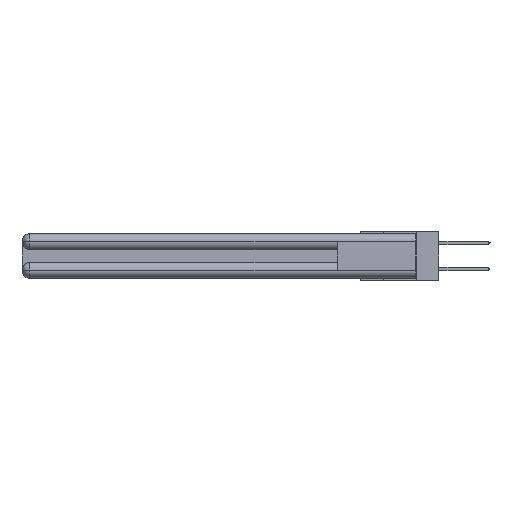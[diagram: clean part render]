
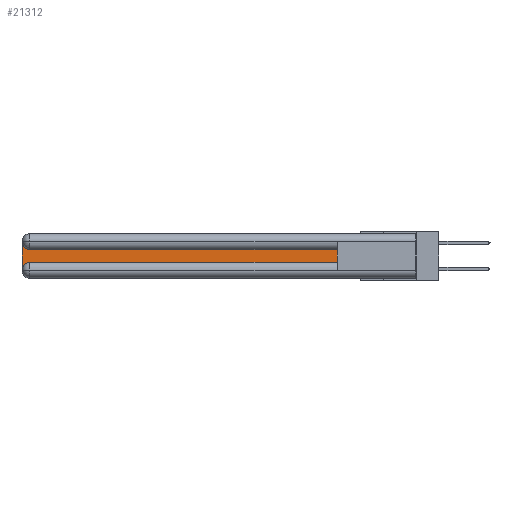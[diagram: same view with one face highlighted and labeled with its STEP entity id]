
A CAD part, left-side view. The second image highlights one B-rep face of the part: STEP entity #21312.
In plain terms, the highlighted planar face has unit normal (-1, 0, 0).
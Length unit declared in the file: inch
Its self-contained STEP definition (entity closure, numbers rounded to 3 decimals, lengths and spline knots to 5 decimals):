
#41 = VERTEX_POINT ( 'NONE', #17808 ) ;
#3055 = CIRCLE ( 'NONE', #13408, 0.06 ) ;
#3262 = VERTEX_POINT ( 'NONE', #27725 ) ;
#3835 = DIRECTION ( 'NONE',  ( 0., 0., -1. ) ) ;
#3892 = EDGE_CURVE ( 'NONE', #3262, #8404, #28747, .T. ) ;
#4001 = ORIENTED_EDGE ( 'NONE', *, *, #3892, .T. ) ;
#4354 = LINE ( 'NONE', #16799, #27396 ) ;
#5309 = DIRECTION ( 'NONE',  ( 0., 0., -1. ) ) ;
#5625 = EDGE_LOOP ( 'NONE', ( #20605, #6453, #24570, #31134, #4001, #34889 ) ) ;
#6453 = ORIENTED_EDGE ( 'NONE', *, *, #14215, .T. ) ;
#8404 = VERTEX_POINT ( 'NONE', #34848 ) ;
#9536 = VECTOR ( 'NONE', #27382, 39.37008 ) ;
#9634 = AXIS2_PLACEMENT_3D ( 'NONE', #31873, #34538, #9685 ) ;
#9685 = DIRECTION ( 'NONE',  ( 0., 0., -1. ) ) ;
#10927 = VERTEX_POINT ( 'NONE', #34252 ) ;
#11731 = CARTESIAN_POINT ( 'NONE',  ( 0.075, 2.94, -0.2775 ) ) ;
#13265 = CARTESIAN_POINT ( 'NONE',  ( 0.075, 0.6, -0.2175 ) ) ;
#13408 = AXIS2_PLACEMENT_3D ( 'NONE', #28506, #25515, #3835 ) ;
#13974 = EDGE_CURVE ( 'NONE', #10927, #41, #4354, .T. ) ;
#14156 = DIRECTION ( 'NONE',  ( 0., 0., 1. ) ) ;
#14215 = EDGE_CURVE ( 'NONE', #41, #34868, #3055, .T. ) ;
#14374 = AXIS2_PLACEMENT_3D ( 'NONE', #11731, #30846, #17394 ) ;
#14524 = LINE ( 'NONE', #18925, #17041 ) ;
#16799 = CARTESIAN_POINT ( 'NONE',  ( 0.075, 0.6, -0.1225 ) ) ;
#17041 = VECTOR ( 'NONE', #5309, 39.37008 ) ;
#17394 = DIRECTION ( 'NONE',  ( 0., 0., -1. ) ) ;
#17808 = CARTESIAN_POINT ( 'NONE',  ( 0.075, 2.94, -0.1225 ) ) ;
#18925 = CARTESIAN_POINT ( 'NONE',  ( 0.075, 3., -0.2175 ) ) ;
#20605 = ORIENTED_EDGE ( 'NONE', *, *, #13974, .T. ) ;
#21067 = CIRCLE ( 'NONE', #14374, 0.06 ) ;
#21312 = ADVANCED_FACE ( 'NONE', ( #34940 ), #34177, .F. ) ;
#23642 = EDGE_CURVE ( 'NONE', #8404, #10927, #28212, .T. ) ;
#24570 = ORIENTED_EDGE ( 'NONE', *, *, #35214, .T. ) ;
#25515 = DIRECTION ( 'NONE',  ( 1., 0., 0. ) ) ;
#27382 = DIRECTION ( 'NONE',  ( 0., -1., 0. ) ) ;
#27396 = VECTOR ( 'NONE', #30708, 39.37008 ) ;
#27725 = CARTESIAN_POINT ( 'NONE',  ( 0.075, 2.94, -0.2175 ) ) ;
#28212 = LINE ( 'NONE', #30882, #34206 ) ;
#28506 = CARTESIAN_POINT ( 'NONE',  ( 0.075, 2.94, -0.0625 ) ) ;
#28747 = LINE ( 'NONE', #13265, #9536 ) ;
#30516 = EDGE_CURVE ( 'NONE', #34157, #3262, #21067, .T. ) ;
#30708 = DIRECTION ( 'NONE',  ( 0., 1., 0. ) ) ;
#30846 = DIRECTION ( 'NONE',  ( 1., 0., 0. ) ) ;
#30882 = CARTESIAN_POINT ( 'NONE',  ( 0.075, 0.6, -0.2175 ) ) ;
#31134 = ORIENTED_EDGE ( 'NONE', *, *, #30516, .T. ) ;
#31534 = CARTESIAN_POINT ( 'NONE',  ( 0.075, 3., -0.0625 ) ) ;
#31873 = CARTESIAN_POINT ( 'NONE',  ( 0.075, 3., -0.1225 ) ) ;
#34100 = CARTESIAN_POINT ( 'NONE',  ( 0.075, 3., -0.2775 ) ) ;
#34157 = VERTEX_POINT ( 'NONE', #34100 ) ;
#34177 = PLANE ( 'NONE',  #9634 ) ;
#34206 = VECTOR ( 'NONE', #14156, 39.37008 ) ;
#34252 = CARTESIAN_POINT ( 'NONE',  ( 0.075, 0.6, -0.1225 ) ) ;
#34538 = DIRECTION ( 'NONE',  ( 1., 0., 0. ) ) ;
#34848 = CARTESIAN_POINT ( 'NONE',  ( 0.075, 0.6, -0.2175 ) ) ;
#34868 = VERTEX_POINT ( 'NONE', #31534 ) ;
#34889 = ORIENTED_EDGE ( 'NONE', *, *, #23642, .T. ) ;
#34940 = FACE_OUTER_BOUND ( 'NONE', #5625, .T. ) ;
#35214 = EDGE_CURVE ( 'NONE', #34868, #34157, #14524, .T. ) ;
